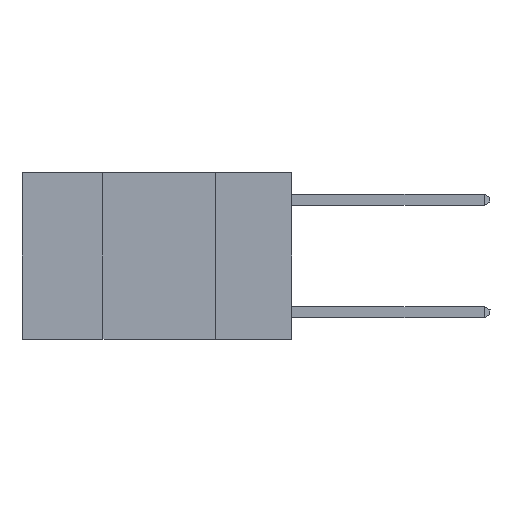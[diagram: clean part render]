
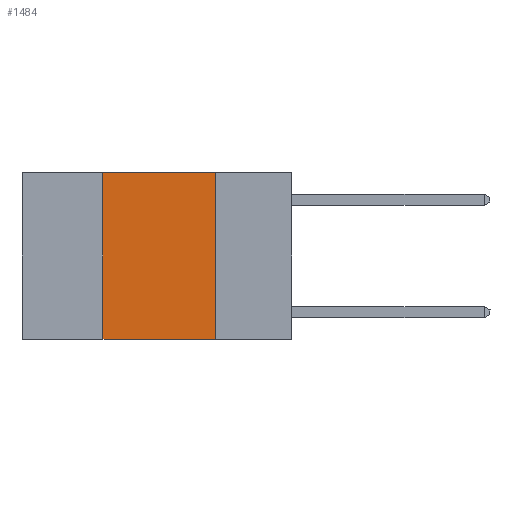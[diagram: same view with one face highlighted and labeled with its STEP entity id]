
A CAD part, left-side view. The second image highlights one B-rep face of the part: STEP entity #1484.
In plain terms, the highlighted planar face has unit normal (-1, 0, 0).
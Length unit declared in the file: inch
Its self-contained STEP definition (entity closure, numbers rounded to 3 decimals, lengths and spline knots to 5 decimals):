
#1081 = VERTEX_POINT ( 'NONE', #5504 ) ;
#1294 = VECTOR ( 'NONE', #5568, 39.37008 ) ;
#1460 = ORIENTED_EDGE ( 'NONE', *, *, #10418, .F. ) ;
#1484 = ADVANCED_FACE ( 'NONE', ( #5128 ), #9483, .F. ) ;
#1597 = ORIENTED_EDGE ( 'NONE', *, *, #6582, .F. ) ;
#1737 = ORIENTED_EDGE ( 'NONE', *, *, #8665, .F. ) ;
#1925 = ORIENTED_EDGE ( 'NONE', *, *, #7178, .T. ) ;
#2118 = VERTEX_POINT ( 'NONE', #6468 ) ;
#2182 = DIRECTION ( 'NONE',  ( 0., -1., 0. ) ) ;
#2455 = VERTEX_POINT ( 'NONE', #9355 ) ;
#2974 = CARTESIAN_POINT ( 'NONE',  ( 0., 0.17, 0. ) ) ;
#3083 = CARTESIAN_POINT ( 'NONE',  ( 0., 0.42, 0. ) ) ;
#4615 = DIRECTION ( 'NONE',  ( 0., 0., -1. ) ) ;
#4742 = LINE ( 'NONE', #5553, #8383 ) ;
#4955 = LINE ( 'NONE', #2974, #6933 ) ;
#5128 = FACE_OUTER_BOUND ( 'NONE', #10554, .T. ) ;
#5346 = DIRECTION ( 'NONE',  ( 0., 0., -1. ) ) ;
#5504 = CARTESIAN_POINT ( 'NONE',  ( 0., 0.42, -0.37 ) ) ;
#5553 = CARTESIAN_POINT ( 'NONE',  ( 0., 0.6, -0.37 ) ) ;
#5568 = DIRECTION ( 'NONE',  ( 0., -1., 0. ) ) ;
#5801 = LINE ( 'NONE', #8072, #1294 ) ;
#6269 = VERTEX_POINT ( 'NONE', #6949 ) ;
#6323 = VECTOR ( 'NONE', #6435, 39.37008 ) ;
#6435 = DIRECTION ( 'NONE',  ( 0., 0., 1. ) ) ;
#6468 = CARTESIAN_POINT ( 'NONE',  ( 0., 0.17, -0.37 ) ) ;
#6582 = EDGE_CURVE ( 'NONE', #2455, #6269, #5801, .T. ) ;
#6933 = VECTOR ( 'NONE', #4615, 39.37008 ) ;
#6949 = CARTESIAN_POINT ( 'NONE',  ( 0., 0.17, 0. ) ) ;
#7178 = EDGE_CURVE ( 'NONE', #1081, #2118, #4742, .T. ) ;
#8072 = CARTESIAN_POINT ( 'NONE',  ( 0., 0.6, 0. ) ) ;
#8383 = VECTOR ( 'NONE', #2182, 39.37008 ) ;
#8498 = LINE ( 'NONE', #3083, #6323 ) ;
#8657 = CARTESIAN_POINT ( 'NONE',  ( 0., 0.6, 0. ) ) ;
#8665 = EDGE_CURVE ( 'NONE', #1081, #2455, #8498, .T. ) ;
#9355 = CARTESIAN_POINT ( 'NONE',  ( 0., 0.42, 0. ) ) ;
#9483 = PLANE ( 'NONE',  #10567 ) ;
#10338 = DIRECTION ( 'NONE',  ( 1., 0., 0. ) ) ;
#10418 = EDGE_CURVE ( 'NONE', #6269, #2118, #4955, .T. ) ;
#10554 = EDGE_LOOP ( 'NONE', ( #1460, #1597, #1737, #1925 ) ) ;
#10567 = AXIS2_PLACEMENT_3D ( 'NONE', #8657, #10338, #5346 ) ;
